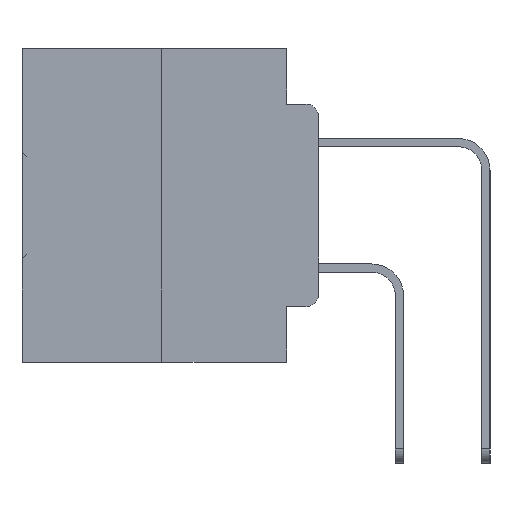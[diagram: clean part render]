
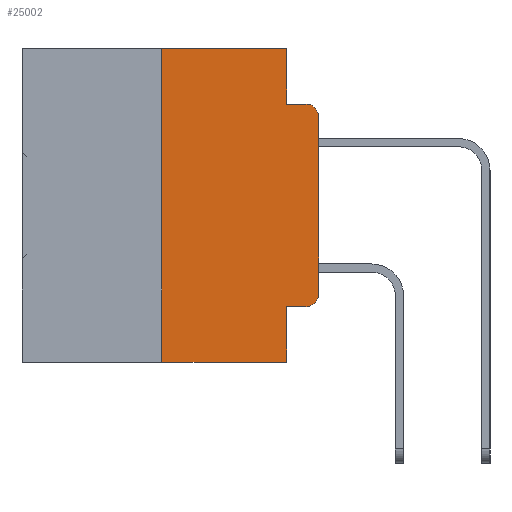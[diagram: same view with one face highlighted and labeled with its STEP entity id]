
A CAD part, left-side view. The second image highlights one B-rep face of the part: STEP entity #25002.
In plain terms, the highlighted planar face has unit normal (-1, 0, 0).
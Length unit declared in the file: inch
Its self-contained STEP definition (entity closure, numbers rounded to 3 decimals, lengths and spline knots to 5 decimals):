
#106 = ORIENTED_EDGE ( 'NONE', *, *, #11730, .T. ) ;
#152 = EDGE_CURVE ( 'NONE', #21812, #32102, #7477, .T. ) ;
#394 = LINE ( 'NONE', #30543, #12267 ) ;
#470 = DIRECTION ( 'NONE',  ( 0., -1., 0. ) ) ;
#562 = VECTOR ( 'NONE', #470, 39.37008 ) ;
#1426 = LINE ( 'NONE', #14027, #562 ) ;
#1676 = DIRECTION ( 'NONE',  ( 0., 0., -1. ) ) ;
#1777 = VERTEX_POINT ( 'NONE', #7819 ) ;
#2120 = DIRECTION ( 'NONE',  ( 1., 0., 0. ) ) ;
#4040 = ORIENTED_EDGE ( 'NONE', *, *, #28214, .T. ) ;
#4452 = ORIENTED_EDGE ( 'NONE', *, *, #30215, .F. ) ;
#5598 = EDGE_CURVE ( 'NONE', #28620, #21812, #8776, .T. ) ;
#5988 = CIRCLE ( 'NONE', #11563, 0.02 ) ;
#7027 = ORIENTED_EDGE ( 'NONE', *, *, #14650, .F. ) ;
#7477 = CIRCLE ( 'NONE', #30911, 0.02 ) ;
#7819 = CARTESIAN_POINT ( 'NONE',  ( 0., 0.051, -0.5 ) ) ;
#8282 = ORIENTED_EDGE ( 'NONE', *, *, #5598, .T. ) ;
#8288 = DIRECTION ( 'NONE',  ( 0., -1., 0. ) ) ;
#8776 = LINE ( 'NONE', #27156, #15184 ) ;
#8961 = VERTEX_POINT ( 'NONE', #19205 ) ;
#8992 = DIRECTION ( 'NONE',  ( 0., -1., 0. ) ) ;
#9062 = CARTESIAN_POINT ( 'NONE',  ( 0., 0.25, 0. ) ) ;
#9145 = EDGE_LOOP ( 'NONE', ( #8282, #15565, #18171, #4452, #7027, #23410, #4040, #18632, #25961, #106 ) ) ;
#9524 = CARTESIAN_POINT ( 'NONE',  ( 0., 0.051, 0. ) ) ;
#11282 = DIRECTION ( 'NONE',  ( 0., -1., 0. ) ) ;
#11563 = AXIS2_PLACEMENT_3D ( 'NONE', #34369, #18041, #1676 ) ;
#11730 = EDGE_CURVE ( 'NONE', #17113, #28620, #5988, .T. ) ;
#11734 = DIRECTION ( 'NONE',  ( 0., 0., -1. ) ) ;
#12267 = VECTOR ( 'NONE', #11282, 39.37008 ) ;
#12686 = CARTESIAN_POINT ( 'NONE',  ( 0., 0., -0.1085 ) ) ;
#13925 = AXIS2_PLACEMENT_3D ( 'NONE', #15709, #2120, #21305 ) ;
#14027 = CARTESIAN_POINT ( 'NONE',  ( 0., 0.051, -0.0885 ) ) ;
#14114 = CARTESIAN_POINT ( 'NONE',  ( 0., 0.02, -0.1085 ) ) ;
#14421 = VECTOR ( 'NONE', #8992, 39.37008 ) ;
#14506 = CARTESIAN_POINT ( 'NONE',  ( 0., 0.02, -0.0885 ) ) ;
#14650 = EDGE_CURVE ( 'NONE', #30710, #32341, #16882, .T. ) ;
#15158 = FACE_OUTER_BOUND ( 'NONE', #9145, .T. ) ;
#15184 = VECTOR ( 'NONE', #21643, 39.37008 ) ;
#15565 = ORIENTED_EDGE ( 'NONE', *, *, #152, .T. ) ;
#15709 = CARTESIAN_POINT ( 'NONE',  ( 0., 0.473, 0. ) ) ;
#16882 = LINE ( 'NONE', #27554, #23418 ) ;
#16892 = DIRECTION ( 'NONE',  ( 0., 0., -1. ) ) ;
#16992 = LINE ( 'NONE', #9062, #17868 ) ;
#17113 = VERTEX_POINT ( 'NONE', #30741 ) ;
#17868 = VECTOR ( 'NONE', #25557, 39.37008 ) ;
#18041 = DIRECTION ( 'NONE',  ( -1., 0., 0. ) ) ;
#18171 = ORIENTED_EDGE ( 'NONE', *, *, #31995, .F. ) ;
#18632 = ORIENTED_EDGE ( 'NONE', *, *, #21043, .F. ) ;
#18899 = LINE ( 'NONE', #9524, #25365 ) ;
#19174 = EDGE_CURVE ( 'NONE', #30836, #17113, #394, .T. ) ;
#19205 = CARTESIAN_POINT ( 'NONE',  ( 0., 0.051, -0.0885 ) ) ;
#21043 = EDGE_CURVE ( 'NONE', #30836, #1777, #18899, .T. ) ;
#21234 = LINE ( 'NONE', #33652, #27685 ) ;
#21305 = DIRECTION ( 'NONE',  ( 0., 0., -1. ) ) ;
#21643 = DIRECTION ( 'NONE',  ( 0., 0., 1. ) ) ;
#21812 = VERTEX_POINT ( 'NONE', #12686 ) ;
#22760 = CARTESIAN_POINT ( 'NONE',  ( 0., 0.473, -0.5 ) ) ;
#22907 = EDGE_CURVE ( 'NONE', #32406, #30710, #16992, .T. ) ;
#23310 = DIRECTION ( 'NONE',  ( 0., 0., -1. ) ) ;
#23410 = ORIENTED_EDGE ( 'NONE', *, *, #22907, .F. ) ;
#23418 = VECTOR ( 'NONE', #8288, 39.37008 ) ;
#23951 = CARTESIAN_POINT ( 'NONE',  ( 0., 0.051, 0. ) ) ;
#25002 = ADVANCED_FACE ( 'NONE', ( #15158 ), #32129, .F. ) ;
#25365 = VECTOR ( 'NONE', #23310, 39.37008 ) ;
#25557 = DIRECTION ( 'NONE',  ( 0., 0., 1. ) ) ;
#25961 = ORIENTED_EDGE ( 'NONE', *, *, #19174, .T. ) ;
#27156 = CARTESIAN_POINT ( 'NONE',  ( 0., 0., 0. ) ) ;
#27554 = CARTESIAN_POINT ( 'NONE',  ( 0., 0.473, 0. ) ) ;
#27685 = VECTOR ( 'NONE', #11734, 39.37008 ) ;
#27785 = CARTESIAN_POINT ( 'NONE',  ( 0., 0.25, 0. ) ) ;
#28214 = EDGE_CURVE ( 'NONE', #32406, #1777, #29114, .T. ) ;
#28620 = VERTEX_POINT ( 'NONE', #30009 ) ;
#29114 = LINE ( 'NONE', #22760, #14421 ) ;
#30009 = CARTESIAN_POINT ( 'NONE',  ( 0., 0., -0.3915 ) ) ;
#30215 = EDGE_CURVE ( 'NONE', #32341, #8961, #21234, .T. ) ;
#30543 = CARTESIAN_POINT ( 'NONE',  ( 0., 0.051, -0.4115 ) ) ;
#30710 = VERTEX_POINT ( 'NONE', #27785 ) ;
#30741 = CARTESIAN_POINT ( 'NONE',  ( 0., 0.02, -0.4115 ) ) ;
#30836 = VERTEX_POINT ( 'NONE', #33613 ) ;
#30911 = AXIS2_PLACEMENT_3D ( 'NONE', #14114, #33267, #16892 ) ;
#31995 = EDGE_CURVE ( 'NONE', #8961, #32102, #1426, .T. ) ;
#32102 = VERTEX_POINT ( 'NONE', #14506 ) ;
#32129 = PLANE ( 'NONE',  #13925 ) ;
#32341 = VERTEX_POINT ( 'NONE', #23951 ) ;
#32406 = VERTEX_POINT ( 'NONE', #34284 ) ;
#33267 = DIRECTION ( 'NONE',  ( -1., 0., 0. ) ) ;
#33613 = CARTESIAN_POINT ( 'NONE',  ( 0., 0.051, -0.4115 ) ) ;
#33652 = CARTESIAN_POINT ( 'NONE',  ( 0., 0.051, 0. ) ) ;
#34284 = CARTESIAN_POINT ( 'NONE',  ( 0., 0.25, -0.5 ) ) ;
#34369 = CARTESIAN_POINT ( 'NONE',  ( 0., 0.02, -0.3915 ) ) ;
